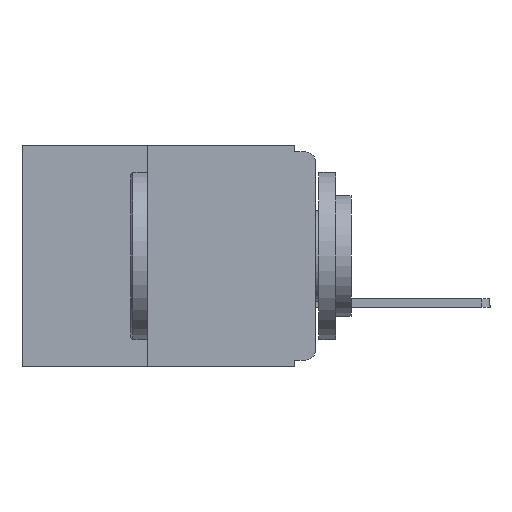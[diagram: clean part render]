
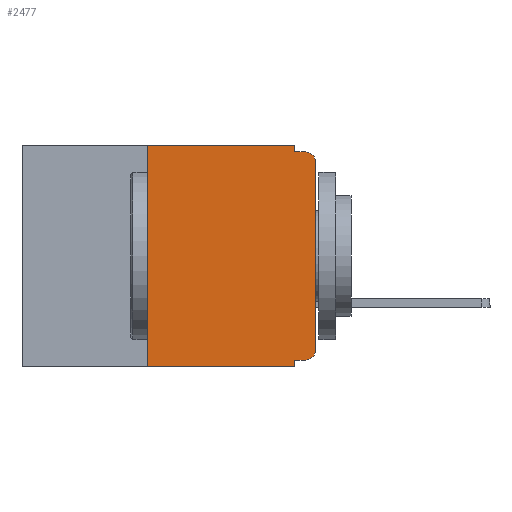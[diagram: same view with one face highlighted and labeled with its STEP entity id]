
A CAD part, left-side view. The second image highlights one B-rep face of the part: STEP entity #2477.
In plain terms, the highlighted planar face has unit normal (-1, 0, 0).
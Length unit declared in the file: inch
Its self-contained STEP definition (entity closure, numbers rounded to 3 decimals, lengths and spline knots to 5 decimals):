
#25 = EDGE_LOOP ( 'NONE', ( #3787, #5604, #6259, #7037, #7406, #7966, #8143, #9719, #10074, #10115 ) ) ;
#274 = AXIS2_PLACEMENT_3D ( 'NONE', #8945, #12636, #5261 ) ;
#426 = VERTEX_POINT ( 'NONE', #12234 ) ;
#463 = VERTEX_POINT ( 'NONE', #19458 ) ;
#1782 = CARTESIAN_POINT ( 'NONE',  ( 0., 0.25, -0.33 ) ) ;
#1857 = EDGE_CURVE ( 'NONE', #15820, #12576, #4639, .T. ) ;
#2030 = EDGE_CURVE ( 'NONE', #463, #14629, #17829, .T. ) ;
#2051 = EDGE_CURVE ( 'NONE', #3704, #426, #18021, .T. ) ;
#2477 = ADVANCED_FACE ( 'NONE', ( #6629 ), #18194, .F. ) ;
#2529 = DIRECTION ( 'NONE',  ( 0., 0., -1. ) ) ;
#2684 = CARTESIAN_POINT ( 'NONE',  ( 0., 0.031, 0. ) ) ;
#3426 = VECTOR ( 'NONE', #11353, 39.37008 ) ;
#3704 = VERTEX_POINT ( 'NONE', #20084 ) ;
#3787 = ORIENTED_EDGE ( 'NONE', *, *, #9195, .T. ) ;
#4025 = VECTOR ( 'NONE', #10355, 39.37008 ) ;
#4068 = LINE ( 'NONE', #10614, #4025 ) ;
#4518 = VECTOR ( 'NONE', #7361, 39.37008 ) ;
#4541 = LINE ( 'NONE', #7365, #4518 ) ;
#4639 = LINE ( 'NONE', #9353, #3426 ) ;
#4992 = CARTESIAN_POINT ( 'NONE',  ( 0., 0.437, 0. ) ) ;
#5261 = DIRECTION ( 'NONE',  ( 0., 0., -1. ) ) ;
#5604 = ORIENTED_EDGE ( 'NONE', *, *, #6082, .T. ) ;
#6082 = EDGE_CURVE ( 'NONE', #17562, #12576, #8701, .T. ) ;
#6259 = ORIENTED_EDGE ( 'NONE', *, *, #1857, .F. ) ;
#6565 = VERTEX_POINT ( 'NONE', #16055 ) ;
#6629 = FACE_OUTER_BOUND ( 'NONE', #25, .T. ) ;
#7037 = ORIENTED_EDGE ( 'NONE', *, *, #16893, .F. ) ;
#7201 = DIRECTION ( 'NONE',  ( 0., 0., -1. ) ) ;
#7277 = CARTESIAN_POINT ( 'NONE',  ( 0., 0., 0. ) ) ;
#7281 = DIRECTION ( 'NONE',  ( -1., 0., 0. ) ) ;
#7361 = DIRECTION ( 'NONE',  ( 0., 0., -1. ) ) ;
#7365 = CARTESIAN_POINT ( 'NONE',  ( 0., 0.031, -0.33 ) ) ;
#7395 = CARTESIAN_POINT ( 'NONE',  ( 0., 0.015, -0.305 ) ) ;
#7406 = ORIENTED_EDGE ( 'NONE', *, *, #2051, .F. ) ;
#7610 = VECTOR ( 'NONE', #2529, 39.37008 ) ;
#7966 = ORIENTED_EDGE ( 'NONE', *, *, #11298, .F. ) ;
#8049 = VECTOR ( 'NONE', #18821, 39.37008 ) ;
#8122 = LINE ( 'NONE', #19210, #8049 ) ;
#8143 = ORIENTED_EDGE ( 'NONE', *, *, #15175, .T. ) ;
#8701 = CIRCLE ( 'NONE', #11784, 0.015 ) ;
#8945 = CARTESIAN_POINT ( 'NONE',  ( 0., 0.437, 0. ) ) ;
#9111 = DIRECTION ( 'NONE',  ( 0., 0., -1. ) ) ;
#9152 = DIRECTION ( 'NONE',  ( -1., 0., 0. ) ) ;
#9186 = CARTESIAN_POINT ( 'NONE',  ( 0., 0.015, -0.025 ) ) ;
#9195 = EDGE_CURVE ( 'NONE', #10836, #17562, #17048, .T. ) ;
#9226 = LINE ( 'NONE', #2684, #7610 ) ;
#9353 = CARTESIAN_POINT ( 'NONE',  ( 0., 0., -0.01 ) ) ;
#9516 = EDGE_CURVE ( 'NONE', #463, #10836, #14405, .T. ) ;
#9719 = ORIENTED_EDGE ( 'NONE', *, *, #17978, .F. ) ;
#10074 = ORIENTED_EDGE ( 'NONE', *, *, #2030, .F. ) ;
#10115 = ORIENTED_EDGE ( 'NONE', *, *, #9516, .T. ) ;
#10354 = CARTESIAN_POINT ( 'NONE',  ( 0., 0., -0.32 ) ) ;
#10355 = DIRECTION ( 'NONE',  ( 0., 0., 1. ) ) ;
#10614 = CARTESIAN_POINT ( 'NONE',  ( 0., 0.25, -0.33 ) ) ;
#10836 = VERTEX_POINT ( 'NONE', #16344 ) ;
#11298 = EDGE_CURVE ( 'NONE', #19687, #3704, #4068, .T. ) ;
#11353 = DIRECTION ( 'NONE',  ( 0., -1., 0. ) ) ;
#11784 = AXIS2_PLACEMENT_3D ( 'NONE', #9186, #9152, #9111 ) ;
#12234 = CARTESIAN_POINT ( 'NONE',  ( 0., 0.031, 0. ) ) ;
#12576 = VERTEX_POINT ( 'NONE', #19428 ) ;
#12636 = DIRECTION ( 'NONE',  ( 1., 0., 0. ) ) ;
#12733 = CARTESIAN_POINT ( 'NONE',  ( 0., 0.031, -0.32 ) ) ;
#13299 = DIRECTION ( 'NONE',  ( 0., 0., 1. ) ) ;
#14405 = CIRCLE ( 'NONE', #18472, 0.015 ) ;
#14629 = VERTEX_POINT ( 'NONE', #12733 ) ;
#15002 = VECTOR ( 'NONE', #17862, 39.37008 ) ;
#15023 = VECTOR ( 'NONE', #18564, 39.37008 ) ;
#15175 = EDGE_CURVE ( 'NONE', #19687, #6565, #8122, .T. ) ;
#15820 = VERTEX_POINT ( 'NONE', #18311 ) ;
#16055 = CARTESIAN_POINT ( 'NONE',  ( 0., 0.031, -0.33 ) ) ;
#16344 = CARTESIAN_POINT ( 'NONE',  ( 0., 0., -0.305 ) ) ;
#16426 = VECTOR ( 'NONE', #13299, 39.37008 ) ;
#16804 = CARTESIAN_POINT ( 'NONE',  ( 0., 0., -0.025 ) ) ;
#16893 = EDGE_CURVE ( 'NONE', #426, #15820, #9226, .T. ) ;
#17048 = LINE ( 'NONE', #7277, #16426 ) ;
#17562 = VERTEX_POINT ( 'NONE', #16804 ) ;
#17829 = LINE ( 'NONE', #10354, #15002 ) ;
#17862 = DIRECTION ( 'NONE',  ( 0., 1., 0. ) ) ;
#17978 = EDGE_CURVE ( 'NONE', #14629, #6565, #4541, .T. ) ;
#18021 = LINE ( 'NONE', #4992, #15023 ) ;
#18194 = PLANE ( 'NONE',  #274 ) ;
#18311 = CARTESIAN_POINT ( 'NONE',  ( 0., 0.031, -0.01 ) ) ;
#18472 = AXIS2_PLACEMENT_3D ( 'NONE', #7395, #7281, #7201 ) ;
#18564 = DIRECTION ( 'NONE',  ( 0., -1., 0. ) ) ;
#18821 = DIRECTION ( 'NONE',  ( 0., -1., 0. ) ) ;
#19210 = CARTESIAN_POINT ( 'NONE',  ( 0., 0.437, -0.33 ) ) ;
#19428 = CARTESIAN_POINT ( 'NONE',  ( 0., 0.015, -0.01 ) ) ;
#19458 = CARTESIAN_POINT ( 'NONE',  ( 0., 0.015, -0.32 ) ) ;
#19687 = VERTEX_POINT ( 'NONE', #1782 ) ;
#20084 = CARTESIAN_POINT ( 'NONE',  ( 0., 0.25, 0. ) ) ;
